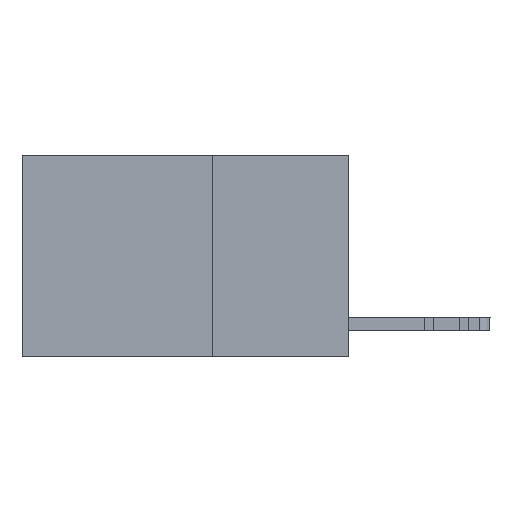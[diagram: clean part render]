
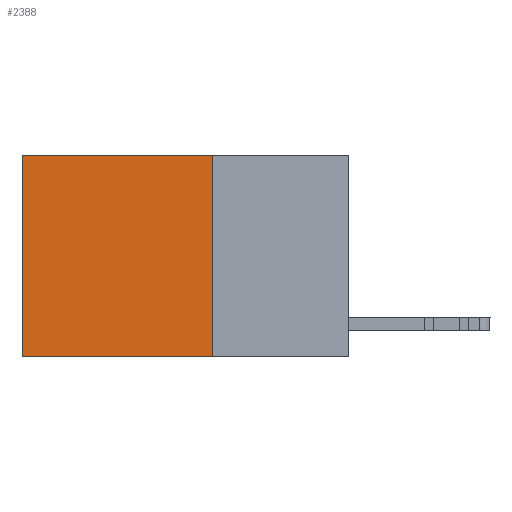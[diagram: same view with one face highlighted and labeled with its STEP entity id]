
A CAD part, left-side view. The second image highlights one B-rep face of the part: STEP entity #2388.
In plain terms, the highlighted planar face has unit normal (-1, 0, 0).
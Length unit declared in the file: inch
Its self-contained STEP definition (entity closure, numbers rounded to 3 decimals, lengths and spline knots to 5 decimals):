
#408 = DIRECTION ( 'NONE',  ( 0., 1., 0. ) ) ;
#1244 = VECTOR ( 'NONE', #25116, 39.37008 ) ;
#1852 = EDGE_CURVE ( 'NONE', #27552, #14308, #16329, .T. ) ;
#2090 = CARTESIAN_POINT ( 'NONE',  ( 0.2625, 0.25, -0.37 ) ) ;
#2388 = ADVANCED_FACE ( 'NONE', ( #23069 ), #10094, .F. ) ;
#3216 = CARTESIAN_POINT ( 'NONE',  ( 0.2625, 0.6, 0. ) ) ;
#3326 = DIRECTION ( 'NONE',  ( 0., 0., -1. ) ) ;
#3356 = ORIENTED_EDGE ( 'NONE', *, *, #18742, .T. ) ;
#3674 = LINE ( 'NONE', #25567, #25916 ) ;
#6769 = VERTEX_POINT ( 'NONE', #2090 ) ;
#6869 = CARTESIAN_POINT ( 'NONE',  ( 0.2625, 0.25, -0.37 ) ) ;
#9943 = VECTOR ( 'NONE', #26538, 39.37008 ) ;
#10094 = PLANE ( 'NONE',  #12756 ) ;
#11118 = EDGE_LOOP ( 'NONE', ( #24904, #12758, #27195, #3356 ) ) ;
#11211 = LINE ( 'NONE', #6869, #27399 ) ;
#12099 = CARTESIAN_POINT ( 'NONE',  ( 0.2625, 0.25, 0. ) ) ;
#12560 = EDGE_CURVE ( 'NONE', #6769, #14308, #11211, .T. ) ;
#12756 = AXIS2_PLACEMENT_3D ( 'NONE', #27671, #19018, #3326 ) ;
#12758 = ORIENTED_EDGE ( 'NONE', *, *, #12560, .F. ) ;
#14308 = VERTEX_POINT ( 'NONE', #24730 ) ;
#15734 = LINE ( 'NONE', #17742, #9943 ) ;
#16329 = LINE ( 'NONE', #3216, #1244 ) ;
#17742 = CARTESIAN_POINT ( 'NONE',  ( 0.2625, 0.25, 0. ) ) ;
#18742 = EDGE_CURVE ( 'NONE', #25937, #27552, #3674, .T. ) ;
#19018 = DIRECTION ( 'NONE',  ( 1., 0., 0. ) ) ;
#21095 = DIRECTION ( 'NONE',  ( 0., 1., 0. ) ) ;
#23069 = FACE_OUTER_BOUND ( 'NONE', #11118, .T. ) ;
#23533 = CARTESIAN_POINT ( 'NONE',  ( 0.2625, 0.6, 0. ) ) ;
#24079 = EDGE_CURVE ( 'NONE', #25937, #6769, #15734, .T. ) ;
#24730 = CARTESIAN_POINT ( 'NONE',  ( 0.2625, 0.6, -0.37 ) ) ;
#24904 = ORIENTED_EDGE ( 'NONE', *, *, #1852, .T. ) ;
#25116 = DIRECTION ( 'NONE',  ( 0., 0., -1. ) ) ;
#25567 = CARTESIAN_POINT ( 'NONE',  ( 0.2625, 0.25, 0. ) ) ;
#25916 = VECTOR ( 'NONE', #21095, 39.37008 ) ;
#25937 = VERTEX_POINT ( 'NONE', #12099 ) ;
#26538 = DIRECTION ( 'NONE',  ( 0., 0., -1. ) ) ;
#27195 = ORIENTED_EDGE ( 'NONE', *, *, #24079, .F. ) ;
#27399 = VECTOR ( 'NONE', #408, 39.37008 ) ;
#27552 = VERTEX_POINT ( 'NONE', #23533 ) ;
#27671 = CARTESIAN_POINT ( 'NONE',  ( 0.2625, 0.25, 0. ) ) ;
